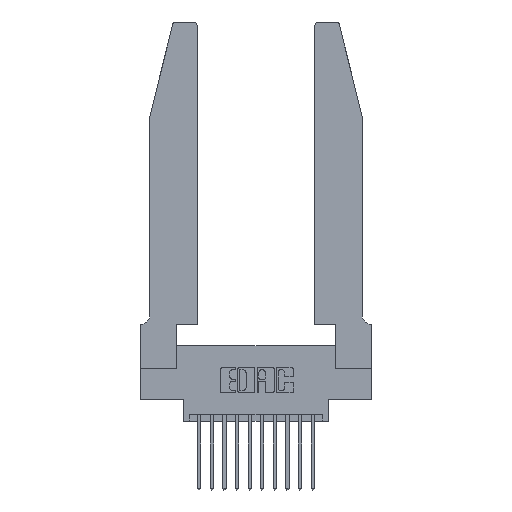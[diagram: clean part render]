
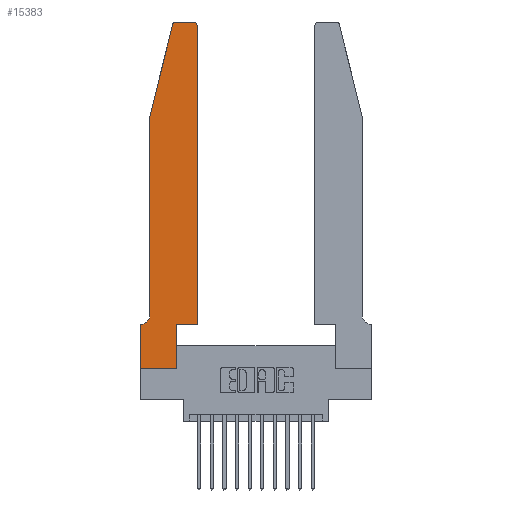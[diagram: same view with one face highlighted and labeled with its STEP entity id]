
A CAD part, top view. The second image highlights one B-rep face of the part: STEP entity #15383.
In plain terms, the highlighted planar face has unit normal (0, 0, 1).
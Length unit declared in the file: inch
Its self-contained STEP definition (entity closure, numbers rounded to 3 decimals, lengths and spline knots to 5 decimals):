
#353 = DIRECTION ( 'NONE',  ( 0., 0., 1. ) ) ;
#417 = VECTOR ( 'NONE', #11176, 39.37008 ) ;
#850 = AXIS2_PLACEMENT_3D ( 'NONE', #3945, #5049, #3715 ) ;
#923 = VERTEX_POINT ( 'NONE', #5793 ) ;
#1025 = CARTESIAN_POINT ( 'NONE',  ( 0.2865, 0., 0.37 ) ) ;
#1128 = CARTESIAN_POINT ( 'NONE',  ( 0.25487, 2.72718, 0.37 ) ) ;
#1340 = ORIENTED_EDGE ( 'NONE', *, *, #11943, .T. ) ;
#1405 = EDGE_CURVE ( 'NONE', #9061, #10782, #5867, .T. ) ;
#1554 = VECTOR ( 'NONE', #14093, 39.37008 ) ;
#1721 = VECTOR ( 'NONE', #13294, 39.37008 ) ;
#1845 = ORIENTED_EDGE ( 'NONE', *, *, #4752, .T. ) ;
#1953 = EDGE_CURVE ( 'NONE', #3995, #923, #10159, .T. ) ;
#1959 = VERTEX_POINT ( 'NONE', #10904 ) ;
#1992 = ORIENTED_EDGE ( 'NONE', *, *, #1405, .T. ) ;
#2314 = VERTEX_POINT ( 'NONE', #8776 ) ;
#2834 = ORIENTED_EDGE ( 'NONE', *, *, #5600, .T. ) ;
#3715 = DIRECTION ( 'NONE',  ( 1., 0., 0. ) ) ;
#3718 = CARTESIAN_POINT ( 'NONE',  ( 0., 0.35, 0.37 ) ) ;
#3923 = VECTOR ( 'NONE', #10033, 39.37008 ) ;
#3931 = VECTOR ( 'NONE', #12679, 39.37008 ) ;
#3945 = CARTESIAN_POINT ( 'NONE',  ( 0.284, 2.72, 0.37 ) ) ;
#3995 = VERTEX_POINT ( 'NONE', #10661 ) ;
#4437 = VERTEX_POINT ( 'NONE', #3718 ) ;
#4539 = EDGE_CURVE ( 'NONE', #10433, #16002, #16001, .T. ) ;
#4704 = DIRECTION ( 'NONE',  ( 0., 1., 0. ) ) ;
#4752 = EDGE_CURVE ( 'NONE', #16002, #15294, #14736, .T. ) ;
#4753 = AXIS2_PLACEMENT_3D ( 'NONE', #11980, #14533, #5423 ) ;
#4802 = ORIENTED_EDGE ( 'NONE', *, *, #4539, .T. ) ;
#4945 = VECTOR ( 'NONE', #10455, 39.37008 ) ;
#5049 = DIRECTION ( 'NONE',  ( 0., 0., 1. ) ) ;
#5331 = ORIENTED_EDGE ( 'NONE', *, *, #14108, .T. ) ;
#5423 = DIRECTION ( 'NONE',  ( 1., 0., 0. ) ) ;
#5600 = EDGE_CURVE ( 'NONE', #11436, #10433, #6290, .T. ) ;
#5793 = CARTESIAN_POINT ( 'NONE',  ( 0.0755, 0.42, 0.37 ) ) ;
#5867 = LINE ( 'NONE', #14890, #10749 ) ;
#5922 = CARTESIAN_POINT ( 'NONE',  ( 0.4505, 2.72, 0.37 ) ) ;
#6290 = CIRCLE ( 'NONE', #8672, 0.03 ) ;
#6472 = VECTOR ( 'NONE', #4704, 39.37008 ) ;
#6595 = ORIENTED_EDGE ( 'NONE', *, *, #7644, .T. ) ;
#6614 = LINE ( 'NONE', #15305, #3923 ) ;
#6832 = EDGE_CURVE ( 'NONE', #923, #1959, #8945, .T. ) ;
#7618 = EDGE_CURVE ( 'NONE', #2314, #9061, #16952, .T. ) ;
#7644 = EDGE_CURVE ( 'NONE', #10782, #15501, #8500, .T. ) ;
#8113 = DIRECTION ( 'NONE',  ( 0., 0., -1. ) ) ;
#8413 = CARTESIAN_POINT ( 'NONE',  ( 0.0755, 0.35, 0.37 ) ) ;
#8500 = LINE ( 'NONE', #10210, #9293 ) ;
#8512 = CARTESIAN_POINT ( 'NONE',  ( 0.2865, 0.35, 0.37 ) ) ;
#8550 = ORIENTED_EDGE ( 'NONE', *, *, #7618, .T. ) ;
#8672 = AXIS2_PLACEMENT_3D ( 'NONE', #14464, #353, #13564 ) ;
#8776 = CARTESIAN_POINT ( 'NONE',  ( 0., 0., 0.37 ) ) ;
#8945 = CIRCLE ( 'NONE', #12178, 0.07 ) ;
#8963 = EDGE_CURVE ( 'NONE', #1959, #4437, #13170, .T. ) ;
#9061 = VERTEX_POINT ( 'NONE', #1025 ) ;
#9293 = VECTOR ( 'NONE', #14154, 39.37008 ) ;
#9297 = PLANE ( 'NONE',  #4753 ) ;
#9569 = CARTESIAN_POINT ( 'NONE',  ( 0.0055, 0.42, 0.37 ) ) ;
#10033 = DIRECTION ( 'NONE',  ( -0.239, -0.971, 0. ) ) ;
#10159 = LINE ( 'NONE', #15436, #1721 ) ;
#10210 = CARTESIAN_POINT ( 'NONE',  ( 0.4505, 0.35, 0.37 ) ) ;
#10433 = VERTEX_POINT ( 'NONE', #15601 ) ;
#10455 = DIRECTION ( 'NONE',  ( 0., -1., 0. ) ) ;
#10644 = ORIENTED_EDGE ( 'NONE', *, *, #6832, .T. ) ;
#10661 = CARTESIAN_POINT ( 'NONE',  ( 0.0755, 2., 0.37 ) ) ;
#10744 = CARTESIAN_POINT ( 'NONE',  ( 0.4505, 0.35, 0.37 ) ) ;
#10749 = VECTOR ( 'NONE', #11884, 39.37008 ) ;
#10782 = VERTEX_POINT ( 'NONE', #8512 ) ;
#10904 = CARTESIAN_POINT ( 'NONE',  ( 0.0055, 0.35, 0.37 ) ) ;
#11176 = DIRECTION ( 'NONE',  ( -1., 0., 0. ) ) ;
#11436 = VERTEX_POINT ( 'NONE', #5922 ) ;
#11875 = EDGE_LOOP ( 'NONE', ( #4802, #1845, #15937, #12518, #10644, #14246, #5331, #8550, #1992, #6595, #1340, #2834 ) ) ;
#11884 = DIRECTION ( 'NONE',  ( 0., 1., 0. ) ) ;
#11943 = EDGE_CURVE ( 'NONE', #15501, #11436, #16354, .T. ) ;
#11980 = CARTESIAN_POINT ( 'NONE',  ( 0., 0.35, 0.37 ) ) ;
#12178 = AXIS2_PLACEMENT_3D ( 'NONE', #9569, #8113, #16188 ) ;
#12518 = ORIENTED_EDGE ( 'NONE', *, *, #1953, .T. ) ;
#12679 = DIRECTION ( 'NONE',  ( 1., 0., 0. ) ) ;
#13170 = LINE ( 'NONE', #8413, #417 ) ;
#13245 = EDGE_CURVE ( 'NONE', #15294, #3995, #6614, .T. ) ;
#13294 = DIRECTION ( 'NONE',  ( 0., -1., 0. ) ) ;
#13564 = DIRECTION ( 'NONE',  ( 1., 0., 0. ) ) ;
#14031 = CARTESIAN_POINT ( 'NONE',  ( 0.2605, 2.75, 0.37 ) ) ;
#14093 = DIRECTION ( 'NONE',  ( -1., 0., 0. ) ) ;
#14108 = EDGE_CURVE ( 'NONE', #4437, #2314, #16914, .T. ) ;
#14154 = DIRECTION ( 'NONE',  ( 1., 0., 0. ) ) ;
#14246 = ORIENTED_EDGE ( 'NONE', *, *, #8963, .T. ) ;
#14464 = CARTESIAN_POINT ( 'NONE',  ( 0.4205, 2.72, 0.37 ) ) ;
#14533 = DIRECTION ( 'NONE',  ( 0., 0., 1. ) ) ;
#14736 = CIRCLE ( 'NONE', #850, 0.03 ) ;
#14890 = CARTESIAN_POINT ( 'NONE',  ( 0.2865, 0.35, 0.37 ) ) ;
#14989 = FACE_OUTER_BOUND ( 'NONE', #11875, .T. ) ;
#15075 = CARTESIAN_POINT ( 'NONE',  ( 0.284, 2.75, 0.37 ) ) ;
#15083 = CARTESIAN_POINT ( 'NONE',  ( 0., 0., 0.37 ) ) ;
#15294 = VERTEX_POINT ( 'NONE', #1128 ) ;
#15305 = CARTESIAN_POINT ( 'NONE',  ( 0.0755, 2., 0.37 ) ) ;
#15309 = CARTESIAN_POINT ( 'NONE',  ( 0.4505, 0.35, 0.37 ) ) ;
#15383 = ADVANCED_FACE ( 'NONE', ( #14989 ), #9297, .T. ) ;
#15436 = CARTESIAN_POINT ( 'NONE',  ( 0.0755, 2., 0.37 ) ) ;
#15501 = VERTEX_POINT ( 'NONE', #10744 ) ;
#15601 = CARTESIAN_POINT ( 'NONE',  ( 0.4205, 2.75, 0.37 ) ) ;
#15851 = CARTESIAN_POINT ( 'NONE',  ( 0., 0., 0.37 ) ) ;
#15937 = ORIENTED_EDGE ( 'NONE', *, *, #13245, .T. ) ;
#16001 = LINE ( 'NONE', #14031, #1554 ) ;
#16002 = VERTEX_POINT ( 'NONE', #15075 ) ;
#16188 = DIRECTION ( 'NONE',  ( -1., 0., 0. ) ) ;
#16354 = LINE ( 'NONE', #15309, #6472 ) ;
#16914 = LINE ( 'NONE', #15851, #4945 ) ;
#16952 = LINE ( 'NONE', #15083, #3931 ) ;
